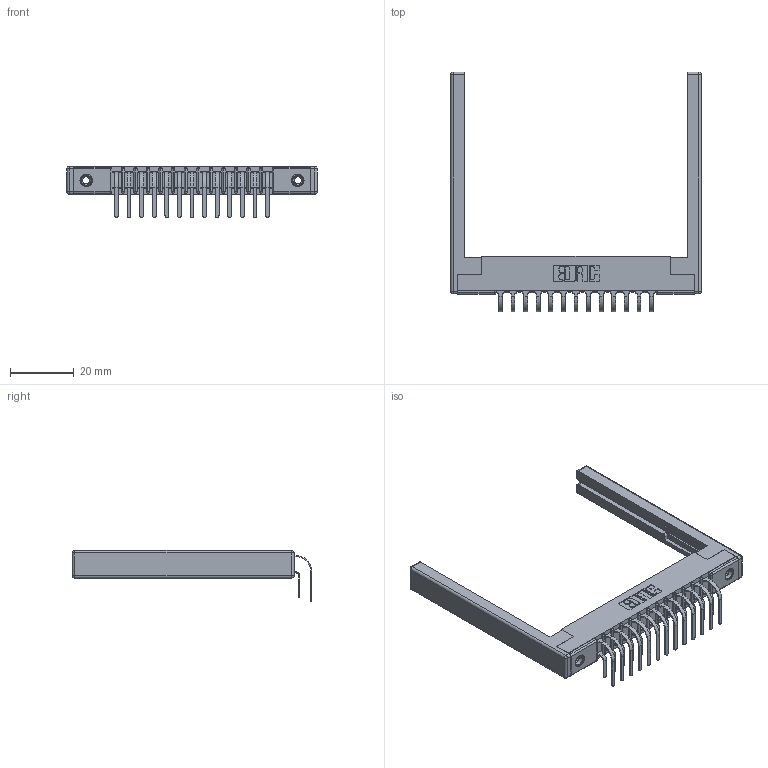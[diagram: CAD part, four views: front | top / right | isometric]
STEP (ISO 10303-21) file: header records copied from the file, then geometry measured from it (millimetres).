
FILE_DESCRIPTION (( 'STEP AP203' ), '1' );
FILE_NAME ('357-026-459-268.STEP', '2022-07-08T00:31:33', ( '' ), ( '' ), 'SwSTEP 2.0', 'SolidWorks 2020', '' );
FILE_SCHEMA (( 'CONFIG_CONTROL_DESIGN' ));
Length unit declared in the file: inch
Products named in the file (6): 307-290-001_558 559 - 1 (Single); 307 Part_.156 Dia Mounting Holes; 345-250-001_345-250-001-102; 357-026-459-268; 307-220-068; 307-290-001_559 - 2 (Single)
Assembly tree (31 placements, depth 2):
  357-026-459-268
    307 Part_.156 Dia Mounting Holes
    307-290-001_558 559 - 1 (Single)  x13
    307-290-001_559 - 2 (Single)  x13
    307-220-068  x2
    345-250-001_345-250-001-102  x2
Bounding box: 78.94 x 75.48 x 16.08 mm (x, y, z)
Volume: 9824 mm3; surface area: 13413.5 mm2
Topology: 31 solids, 31 shells, 1586 faces, 4405 edges, 2842 vertices
Faces by surface type: plane 1016, cylinder 518, sphere 36, cone 12, torus 4
Entity records: 19342 total; most frequent: CARTESIAN_POINT 3152, DIRECTION 3114, ORIENTED_EDGE 3112, EDGE_CURVE 1556, LINE 1178, VECTOR 1178, VERTEX_POINT 1006, AXIS2_PLACEMENT_3D 968
